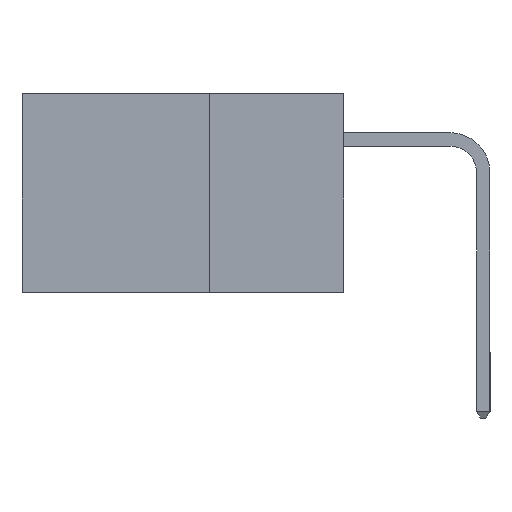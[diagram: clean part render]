
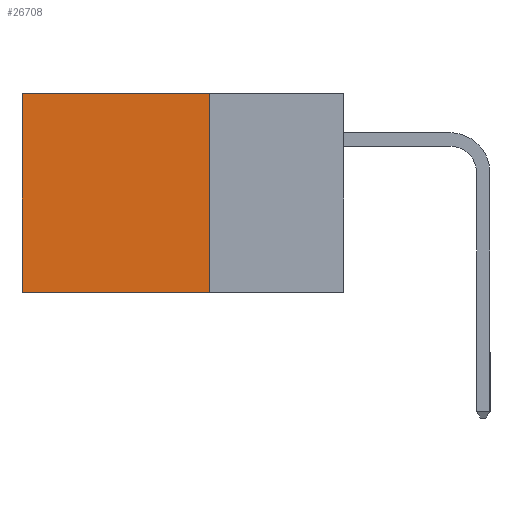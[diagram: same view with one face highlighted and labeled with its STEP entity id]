
A CAD part, left-side view. The second image highlights one B-rep face of the part: STEP entity #26708.
In plain terms, the highlighted planar face has unit normal (-1, 0, 0).
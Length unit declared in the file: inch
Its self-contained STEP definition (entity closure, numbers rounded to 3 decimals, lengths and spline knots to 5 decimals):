
#408 = LINE ( 'NONE', #1327, #17386 ) ;
#1327 = CARTESIAN_POINT ( 'NONE',  ( 0.298, 0.25, 0. ) ) ;
#2849 = CARTESIAN_POINT ( 'NONE',  ( 0.298, 0.6, -0.37 ) ) ;
#4088 = DIRECTION ( 'NONE',  ( 0., 1., 0. ) ) ;
#4510 = VERTEX_POINT ( 'NONE', #20359 ) ;
#5012 = FACE_OUTER_BOUND ( 'NONE', #16953, .T. ) ;
#7062 = EDGE_CURVE ( 'NONE', #11423, #22610, #26054, .T. ) ;
#7331 = ORIENTED_EDGE ( 'NONE', *, *, #26005, .F. ) ;
#9053 = ORIENTED_EDGE ( 'NONE', *, *, #7062, .T. ) ;
#9110 = CARTESIAN_POINT ( 'NONE',  ( 0.298, 0.6, 0. ) ) ;
#10701 = CARTESIAN_POINT ( 'NONE',  ( 0.298, 0.25, -0.37 ) ) ;
#10823 = ORIENTED_EDGE ( 'NONE', *, *, #23132, .F. ) ;
#11423 = VERTEX_POINT ( 'NONE', #9110 ) ;
#12975 = EDGE_CURVE ( 'NONE', #4510, #11423, #19681, .T. ) ;
#13444 = VECTOR ( 'NONE', #18271, 39.37008 ) ;
#13751 = VECTOR ( 'NONE', #18595, 39.37008 ) ;
#15129 = DIRECTION ( 'NONE',  ( 1., 0., 0. ) ) ;
#15693 = LINE ( 'NONE', #10701, #17667 ) ;
#16953 = EDGE_LOOP ( 'NONE', ( #9053, #7331, #10823, #21156 ) ) ;
#17342 = AXIS2_PLACEMENT_3D ( 'NONE', #23391, #15129, #21309 ) ;
#17386 = VECTOR ( 'NONE', #18141, 39.37008 ) ;
#17667 = VECTOR ( 'NONE', #4088, 39.37008 ) ;
#18141 = DIRECTION ( 'NONE',  ( 0., 0., -1. ) ) ;
#18271 = DIRECTION ( 'NONE',  ( 0., 0., -1. ) ) ;
#18595 = DIRECTION ( 'NONE',  ( 0., 1., 0. ) ) ;
#19681 = LINE ( 'NONE', #26887, #13751 ) ;
#20359 = CARTESIAN_POINT ( 'NONE',  ( 0.298, 0.25, 0. ) ) ;
#21156 = ORIENTED_EDGE ( 'NONE', *, *, #12975, .T. ) ;
#21309 = DIRECTION ( 'NONE',  ( 0., 0., -1. ) ) ;
#22288 = VERTEX_POINT ( 'NONE', #26939 ) ;
#22610 = VERTEX_POINT ( 'NONE', #2849 ) ;
#23132 = EDGE_CURVE ( 'NONE', #4510, #22288, #408, .T. ) ;
#23391 = CARTESIAN_POINT ( 'NONE',  ( 0.298, 0.25, 0. ) ) ;
#25622 = PLANE ( 'NONE',  #17342 ) ;
#26005 = EDGE_CURVE ( 'NONE', #22288, #22610, #15693, .T. ) ;
#26054 = LINE ( 'NONE', #26635, #13444 ) ;
#26635 = CARTESIAN_POINT ( 'NONE',  ( 0.298, 0.6, 0. ) ) ;
#26708 = ADVANCED_FACE ( 'NONE', ( #5012 ), #25622, .F. ) ;
#26887 = CARTESIAN_POINT ( 'NONE',  ( 0.298, 0.25, 0. ) ) ;
#26939 = CARTESIAN_POINT ( 'NONE',  ( 0.298, 0.25, -0.37 ) ) ;
